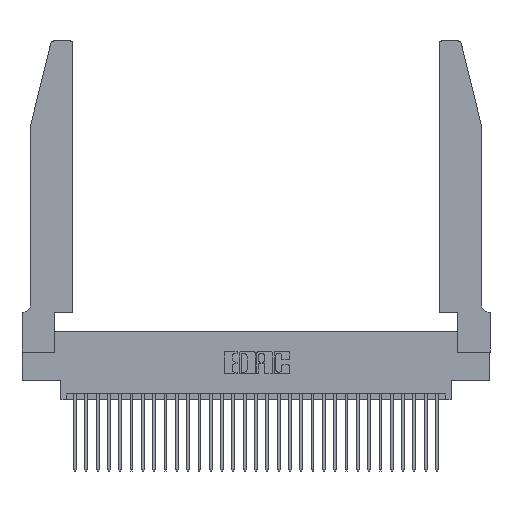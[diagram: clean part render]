
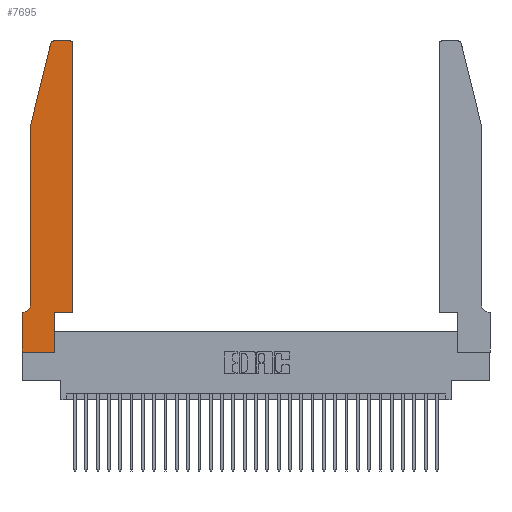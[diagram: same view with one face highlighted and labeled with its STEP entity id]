
A CAD part, top view. The second image highlights one B-rep face of the part: STEP entity #7695.
In plain terms, the highlighted planar face has unit normal (0, 0, 1).
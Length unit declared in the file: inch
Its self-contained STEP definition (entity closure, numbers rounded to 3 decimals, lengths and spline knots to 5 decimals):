
#1636 = ORIENTED_EDGE ( 'NONE', *, *, #12094, .T. ) ;
#1847 = DIRECTION ( 'NONE',  ( 0., 1., 0. ) ) ;
#2228 = CARTESIAN_POINT ( 'NONE',  ( 0.0755, 2., 0.37 ) ) ;
#2326 = CARTESIAN_POINT ( 'NONE',  ( 0.284, 2.75, 0.37 ) ) ;
#2384 = DIRECTION ( 'NONE',  ( 1., 0., 0. ) ) ;
#3175 = AXIS2_PLACEMENT_3D ( 'NONE', #31940, #17336, #2384 ) ;
#3408 = EDGE_CURVE ( 'NONE', #14979, #17561, #22983, .T. ) ;
#4087 = CARTESIAN_POINT ( 'NONE',  ( 0.25487, 2.72718, 0.37 ) ) ;
#4153 = VERTEX_POINT ( 'NONE', #13100 ) ;
#5038 = VECTOR ( 'NONE', #29472, 39.37008 ) ;
#5491 = LINE ( 'NONE', #29507, #23654 ) ;
#5839 = LINE ( 'NONE', #2228, #5038 ) ;
#5912 = CARTESIAN_POINT ( 'NONE',  ( 0.2865, 0., 0.37 ) ) ;
#6317 = AXIS2_PLACEMENT_3D ( 'NONE', #14956, #31991, #17389 ) ;
#6336 = CARTESIAN_POINT ( 'NONE',  ( 0., 0., 0.37 ) ) ;
#7534 = EDGE_CURVE ( 'NONE', #26772, #13166, #10954, .T. ) ;
#7540 = DIRECTION ( 'NONE',  ( -1., 0., 0. ) ) ;
#7603 = VECTOR ( 'NONE', #16338, 39.37008 ) ;
#7695 = ADVANCED_FACE ( 'NONE', ( #12907 ), #8083, .T. ) ;
#7818 = ORIENTED_EDGE ( 'NONE', *, *, #12195, .T. ) ;
#8083 = PLANE ( 'NONE',  #23125 ) ;
#8151 = LINE ( 'NONE', #23366, #27728 ) ;
#8362 = CARTESIAN_POINT ( 'NONE',  ( 0.4505, 2.72, 0.37 ) ) ;
#8496 = VERTEX_POINT ( 'NONE', #2326 ) ;
#8685 = DIRECTION ( 'NONE',  ( 1., 0., 0. ) ) ;
#9002 = ORIENTED_EDGE ( 'NONE', *, *, #29903, .T. ) ;
#9055 = VERTEX_POINT ( 'NONE', #9735 ) ;
#9735 = CARTESIAN_POINT ( 'NONE',  ( 0.4505, 0.35, 0.37 ) ) ;
#10566 = DIRECTION ( 'NONE',  ( 0., 0., 1. ) ) ;
#10954 = CIRCLE ( 'NONE', #3175, 0.03 ) ;
#10966 = CARTESIAN_POINT ( 'NONE',  ( 0.2865, 0.35, 0.37 ) ) ;
#11461 = LINE ( 'NONE', #27289, #25287 ) ;
#12094 = EDGE_CURVE ( 'NONE', #18843, #29515, #12659, .T. ) ;
#12195 = EDGE_CURVE ( 'NONE', #17561, #4153, #29859, .T. ) ;
#12315 = ORIENTED_EDGE ( 'NONE', *, *, #28912, .T. ) ;
#12406 = LINE ( 'NONE', #26786, #31138 ) ;
#12638 = DIRECTION ( 'NONE',  ( 0., -1., 0. ) ) ;
#12659 = LINE ( 'NONE', #14691, #25684 ) ;
#12907 = FACE_OUTER_BOUND ( 'NONE', #19407, .T. ) ;
#12932 = DIRECTION ( 'NONE',  ( 0., 0., -1. ) ) ;
#13008 = ORIENTED_EDGE ( 'NONE', *, *, #7534, .T. ) ;
#13066 = CARTESIAN_POINT ( 'NONE',  ( 0.0755, 0.42, 0.37 ) ) ;
#13100 = CARTESIAN_POINT ( 'NONE',  ( 0., 0.35, 0.37 ) ) ;
#13166 = VERTEX_POINT ( 'NONE', #30448 ) ;
#14487 = DIRECTION ( 'NONE',  ( 0., 1., 0. ) ) ;
#14691 = CARTESIAN_POINT ( 'NONE',  ( 0.0755, 2., 0.37 ) ) ;
#14956 = CARTESIAN_POINT ( 'NONE',  ( 0.284, 2.72, 0.37 ) ) ;
#14979 = VERTEX_POINT ( 'NONE', #13066 ) ;
#16109 = VECTOR ( 'NONE', #7540, 39.37008 ) ;
#16338 = DIRECTION ( 'NONE',  ( 1., 0., 0. ) ) ;
#17333 = DIRECTION ( 'NONE',  ( -1., 0., 0. ) ) ;
#17336 = DIRECTION ( 'NONE',  ( 0., 0., 1. ) ) ;
#17389 = DIRECTION ( 'NONE',  ( 1., 0., 0. ) ) ;
#17561 = VERTEX_POINT ( 'NONE', #20555 ) ;
#18642 = ORIENTED_EDGE ( 'NONE', *, *, #31281, .T. ) ;
#18843 = VERTEX_POINT ( 'NONE', #4087 ) ;
#19407 = EDGE_LOOP ( 'NONE', ( #18642, #21191, #1636, #24906, #29013, #7818, #9002, #12315, #31479, #22939, #29127, #13008 ) ) ;
#20555 = CARTESIAN_POINT ( 'NONE',  ( 0.0055, 0.35, 0.37 ) ) ;
#21191 = ORIENTED_EDGE ( 'NONE', *, *, #26599, .T. ) ;
#21251 = VERTEX_POINT ( 'NONE', #10966 ) ;
#21594 = CARTESIAN_POINT ( 'NONE',  ( 0., 0., 0.37 ) ) ;
#22210 = LINE ( 'NONE', #6336, #7603 ) ;
#22939 = ORIENTED_EDGE ( 'NONE', *, *, #26841, .T. ) ;
#22983 = CIRCLE ( 'NONE', #30873, 0.07 ) ;
#23125 = AXIS2_PLACEMENT_3D ( 'NONE', #25266, #10566, #27718 ) ;
#23366 = CARTESIAN_POINT ( 'NONE',  ( 0.4505, 0.35, 0.37 ) ) ;
#23494 = EDGE_CURVE ( 'NONE', #9055, #26772, #12406, .T. ) ;
#23654 = VECTOR ( 'NONE', #17333, 39.37008 ) ;
#24413 = VERTEX_POINT ( 'NONE', #5912 ) ;
#24906 = ORIENTED_EDGE ( 'NONE', *, *, #31929, .T. ) ;
#25266 = CARTESIAN_POINT ( 'NONE',  ( 0., 0.35, 0.37 ) ) ;
#25287 = VECTOR ( 'NONE', #12638, 39.37008 ) ;
#25684 = VECTOR ( 'NONE', #31737, 39.37008 ) ;
#26030 = CARTESIAN_POINT ( 'NONE',  ( 0.0755, 2., 0.37 ) ) ;
#26599 = EDGE_CURVE ( 'NONE', #8496, #18843, #30198, .T. ) ;
#26772 = VERTEX_POINT ( 'NONE', #8362 ) ;
#26786 = CARTESIAN_POINT ( 'NONE',  ( 0.4505, 0.35, 0.37 ) ) ;
#26841 = EDGE_CURVE ( 'NONE', #21251, #9055, #8151, .T. ) ;
#27071 = EDGE_CURVE ( 'NONE', #24413, #21251, #28097, .T. ) ;
#27197 = CARTESIAN_POINT ( 'NONE',  ( 0.0755, 0.35, 0.37 ) ) ;
#27289 = CARTESIAN_POINT ( 'NONE',  ( 0., 0., 0.37 ) ) ;
#27552 = VERTEX_POINT ( 'NONE', #21594 ) ;
#27580 = CARTESIAN_POINT ( 'NONE',  ( 0.0055, 0.42, 0.37 ) ) ;
#27718 = DIRECTION ( 'NONE',  ( 1., 0., 0. ) ) ;
#27728 = VECTOR ( 'NONE', #8685, 39.37008 ) ;
#28097 = LINE ( 'NONE', #31426, #28832 ) ;
#28832 = VECTOR ( 'NONE', #1847, 39.37008 ) ;
#28912 = EDGE_CURVE ( 'NONE', #27552, #24413, #22210, .T. ) ;
#29013 = ORIENTED_EDGE ( 'NONE', *, *, #3408, .T. ) ;
#29127 = ORIENTED_EDGE ( 'NONE', *, *, #23494, .T. ) ;
#29472 = DIRECTION ( 'NONE',  ( 0., -1., 0. ) ) ;
#29507 = CARTESIAN_POINT ( 'NONE',  ( 0.2605, 2.75, 0.37 ) ) ;
#29515 = VERTEX_POINT ( 'NONE', #26030 ) ;
#29859 = LINE ( 'NONE', #27197, #16109 ) ;
#29903 = EDGE_CURVE ( 'NONE', #4153, #27552, #11461, .T. ) ;
#30014 = DIRECTION ( 'NONE',  ( -1., 0., 0. ) ) ;
#30198 = CIRCLE ( 'NONE', #6317, 0.03 ) ;
#30448 = CARTESIAN_POINT ( 'NONE',  ( 0.4205, 2.75, 0.37 ) ) ;
#30873 = AXIS2_PLACEMENT_3D ( 'NONE', #27580, #12932, #30014 ) ;
#31138 = VECTOR ( 'NONE', #14487, 39.37008 ) ;
#31281 = EDGE_CURVE ( 'NONE', #13166, #8496, #5491, .T. ) ;
#31426 = CARTESIAN_POINT ( 'NONE',  ( 0.2865, 0.35, 0.37 ) ) ;
#31479 = ORIENTED_EDGE ( 'NONE', *, *, #27071, .T. ) ;
#31737 = DIRECTION ( 'NONE',  ( -0.239, -0.971, 0. ) ) ;
#31929 = EDGE_CURVE ( 'NONE', #29515, #14979, #5839, .T. ) ;
#31940 = CARTESIAN_POINT ( 'NONE',  ( 0.4205, 2.72, 0.37 ) ) ;
#31991 = DIRECTION ( 'NONE',  ( 0., 0., 1. ) ) ;
